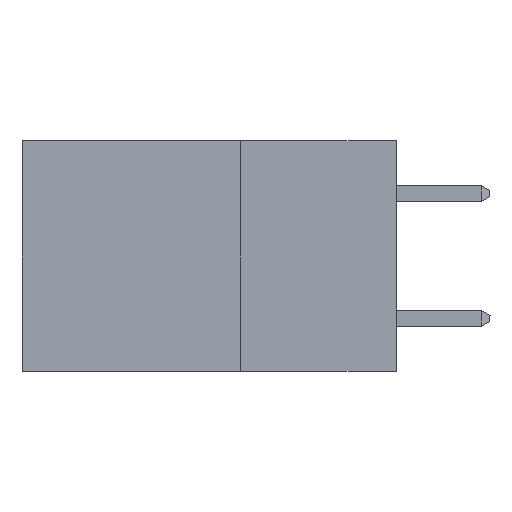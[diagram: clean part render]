
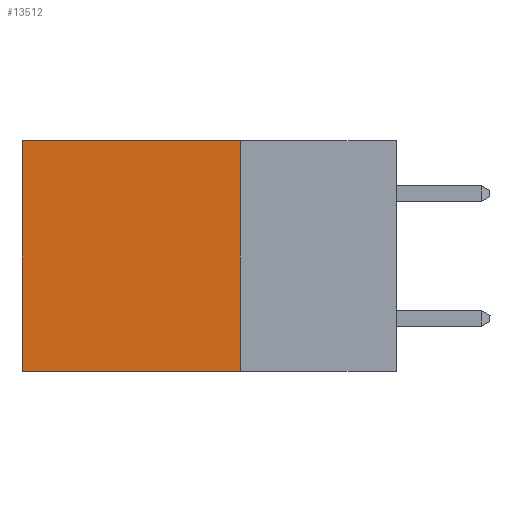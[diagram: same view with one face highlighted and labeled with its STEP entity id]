
A CAD part, left-side view. The second image highlights one B-rep face of the part: STEP entity #13512.
In plain terms, the highlighted planar face has unit normal (-1, 0, 0).
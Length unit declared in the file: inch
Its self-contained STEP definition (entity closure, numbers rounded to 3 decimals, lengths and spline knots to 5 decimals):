
#13 = EDGE_CURVE ( 'NONE', #21163, #12584, #17956, .T. ) ;
#738 = CARTESIAN_POINT ( 'NONE',  ( 0.2615, 0.25, -0.37 ) ) ;
#821 = ORIENTED_EDGE ( 'NONE', *, *, #14840, .T. ) ;
#974 = DIRECTION ( 'NONE',  ( 0., 0., -1. ) ) ;
#1787 = DIRECTION ( 'NONE',  ( 0., 0., -1. ) ) ;
#1824 = CARTESIAN_POINT ( 'NONE',  ( 0.2615, 0.25, -0.37 ) ) ;
#1912 = DIRECTION ( 'NONE',  ( 0., 1., 0. ) ) ;
#2358 = CARTESIAN_POINT ( 'NONE',  ( 0.2615, 0.25, -0.37 ) ) ;
#3526 = ORIENTED_EDGE ( 'NONE', *, *, #6603, .F. ) ;
#3759 = EDGE_CURVE ( 'NONE', #10170, #10969, #13537, .T. ) ;
#6198 = CARTESIAN_POINT ( 'NONE',  ( 0.2615, 0.6, 0. ) ) ;
#6603 = EDGE_CURVE ( 'NONE', #21163, #10170, #8860, .T. ) ;
#6860 = PLANE ( 'NONE',  #10404 ) ;
#7627 = VECTOR ( 'NONE', #1912, 39.37008 ) ;
#8565 = FACE_OUTER_BOUND ( 'NONE', #23108, .T. ) ;
#8860 = LINE ( 'NONE', #1824, #24398 ) ;
#10170 = VERTEX_POINT ( 'NONE', #21197 ) ;
#10404 = AXIS2_PLACEMENT_3D ( 'NONE', #738, #22576, #10844 ) ;
#10844 = DIRECTION ( 'NONE',  ( 0., 0., -1. ) ) ;
#10969 = VERTEX_POINT ( 'NONE', #19470 ) ;
#12207 = DIRECTION ( 'NONE',  ( 0., 1., 0. ) ) ;
#12584 = VERTEX_POINT ( 'NONE', #6198 ) ;
#12744 = VECTOR ( 'NONE', #12207, 39.37008 ) ;
#12985 = CARTESIAN_POINT ( 'NONE',  ( 0.2615, 0.6, -0.37 ) ) ;
#13512 = ADVANCED_FACE ( 'NONE', ( #8565 ), #6860, .F. ) ;
#13537 = LINE ( 'NONE', #2358, #7627 ) ;
#14840 = EDGE_CURVE ( 'NONE', #12584, #10969, #23479, .T. ) ;
#15054 = ORIENTED_EDGE ( 'NONE', *, *, #3759, .F. ) ;
#15239 = ORIENTED_EDGE ( 'NONE', *, *, #13, .T. ) ;
#17956 = LINE ( 'NONE', #21566, #12744 ) ;
#19470 = CARTESIAN_POINT ( 'NONE',  ( 0.2615, 0.6, -0.37 ) ) ;
#19579 = VECTOR ( 'NONE', #974, 39.37008 ) ;
#21163 = VERTEX_POINT ( 'NONE', #21563 ) ;
#21197 = CARTESIAN_POINT ( 'NONE',  ( 0.2615, 0.25, -0.37 ) ) ;
#21563 = CARTESIAN_POINT ( 'NONE',  ( 0.2615, 0.25, 0. ) ) ;
#21566 = CARTESIAN_POINT ( 'NONE',  ( 0.2615, 0.25, 0. ) ) ;
#22576 = DIRECTION ( 'NONE',  ( 1., 0., 0. ) ) ;
#23108 = EDGE_LOOP ( 'NONE', ( #821, #15054, #3526, #15239 ) ) ;
#23479 = LINE ( 'NONE', #12985, #19579 ) ;
#24398 = VECTOR ( 'NONE', #1787, 39.37008 ) ;
